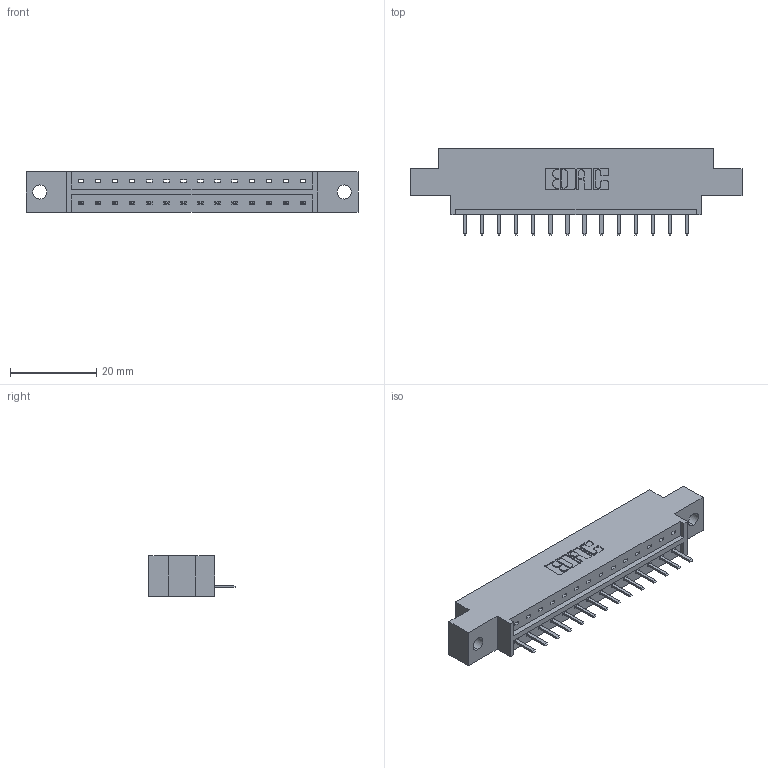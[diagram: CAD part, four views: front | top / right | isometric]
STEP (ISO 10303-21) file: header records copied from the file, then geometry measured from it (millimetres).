
FILE_DESCRIPTION (( 'STEP AP203' ), '1' );
FILE_NAME ('833-014-520-602.STEP', '2020-05-31T01:03:43', ( '' ), ( '' ), 'SwSTEP 2.0', 'SolidWorks 2020', '' );
FILE_SCHEMA (( 'CONFIG_CONTROL_DESIGN' ));
Length unit declared in the file: inch
Products named in the file (3): 833-014-520-602; 833 Part_Offset - .128 Dia; 345-292-001_345-293-120
Assembly tree (15 placements, depth 2):
  833-014-520-602
    833 Part_Offset - .128 Dia
    345-292-001_345-293-120  x14
Bounding box: 77.01 x 20.02 x 9.4 mm (x, y, z)
Volume: 7204.1 mm3; surface area: 7395.9 mm2
Topology: 15 solids, 15 shells, 986 faces, 2899 edges, 1894 vertices
Faces by surface type: plane 690, cylinder 296
Entity records: 12429 total; most frequent: CARTESIAN_POINT 2168, ORIENTED_EDGE 2106, DIRECTION 1873, EDGE_CURVE 1053, VECTOR 921, LINE 921, VERTEX_POINT 698, AXIS2_PLACEMENT_3D 476
